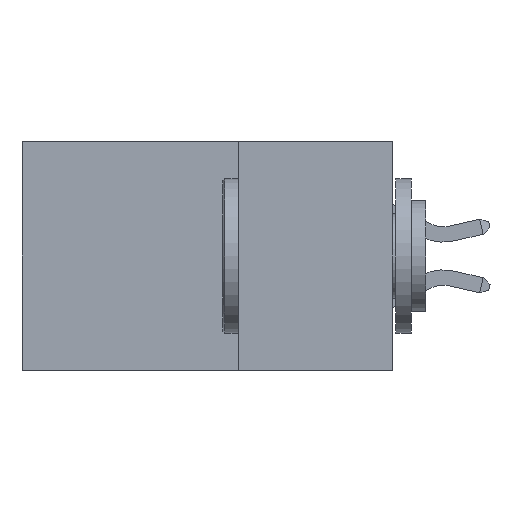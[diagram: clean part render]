
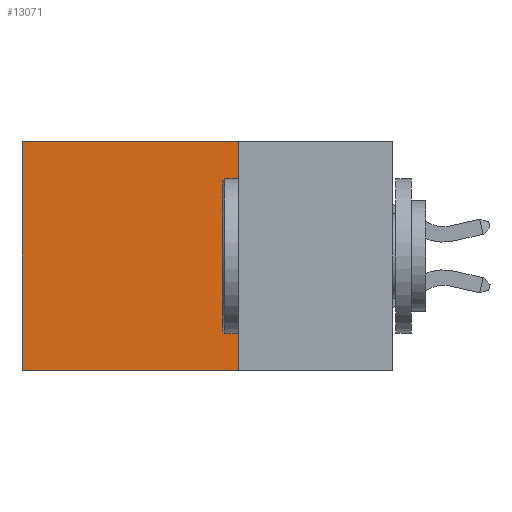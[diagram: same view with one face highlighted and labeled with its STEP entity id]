
A CAD part, left-side view. The second image highlights one B-rep face of the part: STEP entity #13071.
In plain terms, the highlighted planar face has unit normal (-1, 0, 0).
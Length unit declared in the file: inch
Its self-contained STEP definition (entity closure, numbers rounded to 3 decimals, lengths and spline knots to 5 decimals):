
#191 = EDGE_CURVE ( 'NONE', #17398, #17451, #6022, .T. ) ;
#959 = VECTOR ( 'NONE', #5599, 39.37008 ) ;
#1181 = EDGE_CURVE ( 'NONE', #5704, #15934, #12514, .T. ) ;
#1505 = LINE ( 'NONE', #3814, #959 ) ;
#2141 = AXIS2_PLACEMENT_3D ( 'NONE', #20715, #10286, #22431 ) ;
#2826 = LINE ( 'NONE', #20966, #20870 ) ;
#3185 = VECTOR ( 'NONE', #12308, 39.37008 ) ;
#3814 = CARTESIAN_POINT ( 'NONE',  ( 0.2875, 0.6, 0. ) ) ;
#4071 = DIRECTION ( 'NONE',  ( 0., 1., 0. ) ) ;
#4538 = ORIENTED_EDGE ( 'NONE', *, *, #191, .T. ) ;
#5029 = PLANE ( 'NONE',  #2141 ) ;
#5467 = VECTOR ( 'NONE', #4071, 39.37008 ) ;
#5599 = DIRECTION ( 'NONE',  ( 0., 0., -1. ) ) ;
#5704 = VERTEX_POINT ( 'NONE', #8429 ) ;
#6022 = LINE ( 'NONE', #20071, #5467 ) ;
#6478 = EDGE_CURVE ( 'NONE', #17398, #5704, #2826, .T. ) ;
#7381 = EDGE_LOOP ( 'NONE', ( #9420, #22349, #9311, #4538 ) ) ;
#8429 = CARTESIAN_POINT ( 'NONE',  ( 0.2875, 0.25, -0.37 ) ) ;
#8815 = CARTESIAN_POINT ( 'NONE',  ( 0.2875, 0.25, -0.37 ) ) ;
#9311 = ORIENTED_EDGE ( 'NONE', *, *, #6478, .F. ) ;
#9420 = ORIENTED_EDGE ( 'NONE', *, *, #10511, .T. ) ;
#9548 = CARTESIAN_POINT ( 'NONE',  ( 0.2875, 0.25, 0. ) ) ;
#10286 = DIRECTION ( 'NONE',  ( 1., 0., 0. ) ) ;
#10511 = EDGE_CURVE ( 'NONE', #17451, #15934, #1505, .T. ) ;
#12308 = DIRECTION ( 'NONE',  ( 0., 1., 0. ) ) ;
#12514 = LINE ( 'NONE', #8815, #3185 ) ;
#13071 = ADVANCED_FACE ( 'NONE', ( #17724 ), #5029, .F. ) ;
#13190 = CARTESIAN_POINT ( 'NONE',  ( 0.2875, 0.6, 0. ) ) ;
#15934 = VERTEX_POINT ( 'NONE', #16484 ) ;
#16484 = CARTESIAN_POINT ( 'NONE',  ( 0.2875, 0.6, -0.37 ) ) ;
#17398 = VERTEX_POINT ( 'NONE', #9548 ) ;
#17451 = VERTEX_POINT ( 'NONE', #13190 ) ;
#17724 = FACE_OUTER_BOUND ( 'NONE', #7381, .T. ) ;
#20071 = CARTESIAN_POINT ( 'NONE',  ( 0.2875, 0.25, 0. ) ) ;
#20715 = CARTESIAN_POINT ( 'NONE',  ( 0.2875, 0.25, 0. ) ) ;
#20870 = VECTOR ( 'NONE', #22675, 39.37008 ) ;
#20966 = CARTESIAN_POINT ( 'NONE',  ( 0.2875, 0.25, 0. ) ) ;
#22349 = ORIENTED_EDGE ( 'NONE', *, *, #1181, .F. ) ;
#22431 = DIRECTION ( 'NONE',  ( 0., 0., -1. ) ) ;
#22675 = DIRECTION ( 'NONE',  ( 0., 0., -1. ) ) ;
